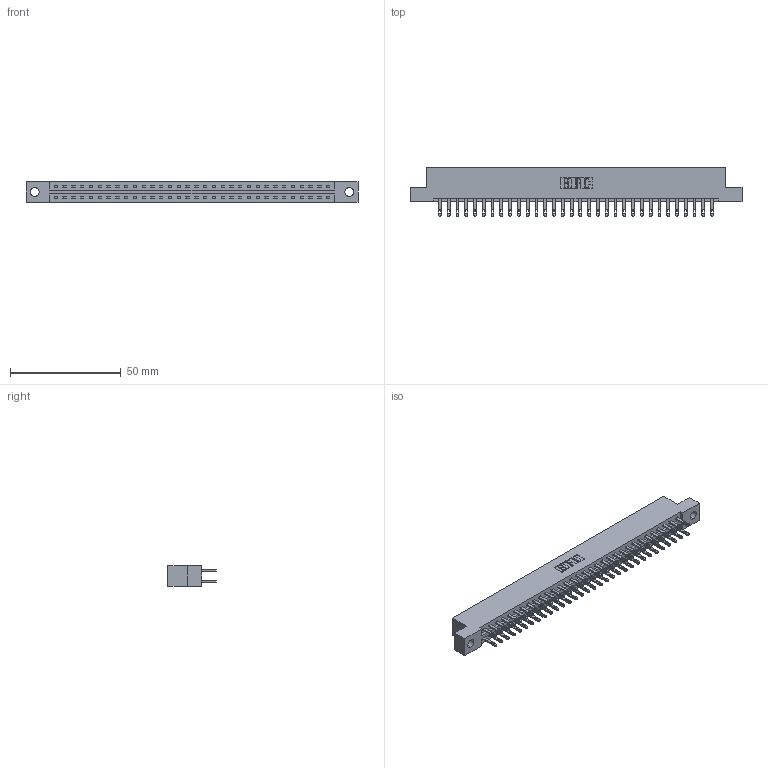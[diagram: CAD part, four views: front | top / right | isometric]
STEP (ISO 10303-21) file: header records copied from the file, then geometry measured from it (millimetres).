
FILE_DESCRIPTION (( 'STEP AP203' ), '1' );
FILE_NAME ('337-064-500-204.STEP', '2019-10-09T21:51:35', ( '' ), ( '' ), 'SwSTEP 2.0', 'SolidWorks 2016', '' );
FILE_SCHEMA (( 'CONFIG_CONTROL_DESIGN' ));
Length unit declared in the file: inch
Products named in the file (3): 345-292-001_345-293-100; 337-064-500-204; 337 Part_Flush Mounting Lugs - 0.156 Dia-TH
Assembly tree (65 placements, depth 2):
  337-064-500-204
    337 Part_Flush Mounting Lugs - 0.156 Dia-TH
    345-292-001_345-293-100  x64
Bounding box: 149.81 x 21.85 x 9.4 mm (x, y, z)
Volume: 15762.7 mm3; surface area: 18230.1 mm2
Topology: 65 solids, 65 shells, 3314 faces, 10103 edges, 6734 vertices
Faces by surface type: plane 2118, cylinder 1196
Entity records: 26037 total; most frequent: CARTESIAN_POINT 4394, ORIENTED_EDGE 4330, DIRECTION 3757, EDGE_CURVE 2165, LINE 2033, VECTOR 2033, VERTEX_POINT 1442, AXIS2_PLACEMENT_3D 862
